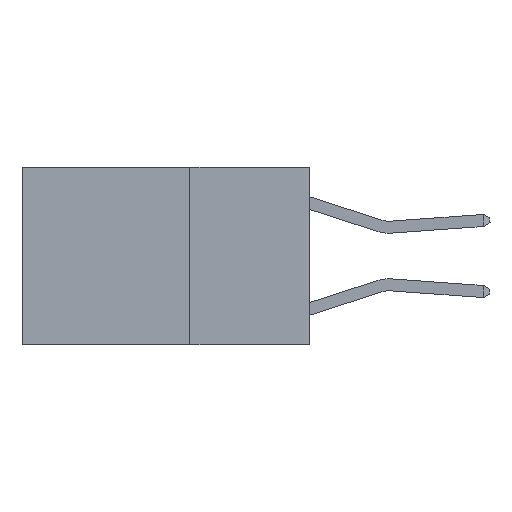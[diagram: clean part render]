
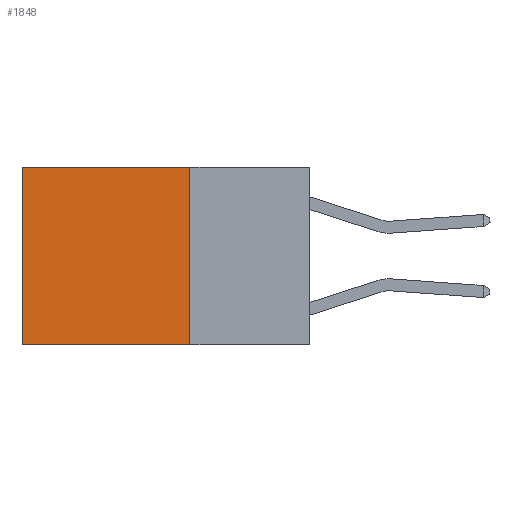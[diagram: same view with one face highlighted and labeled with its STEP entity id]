
A CAD part, left-side view. The second image highlights one B-rep face of the part: STEP entity #1848.
In plain terms, the highlighted planar face has unit normal (-1, 0, 0).
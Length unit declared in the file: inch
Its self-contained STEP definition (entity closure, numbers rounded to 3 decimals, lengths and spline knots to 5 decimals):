
#66 = LINE ( 'NONE', #4859, #17394 ) ;
#236 = LINE ( 'NONE', #1767, #18841 ) ;
#799 = CARTESIAN_POINT ( 'NONE',  ( 0.2625, 0.25, 0. ) ) ;
#1332 = FACE_OUTER_BOUND ( 'NONE', #15989, .T. ) ;
#1666 = ORIENTED_EDGE ( 'NONE', *, *, #2875, .T. ) ;
#1767 = CARTESIAN_POINT ( 'NONE',  ( 0.2625, 0.6, 0. ) ) ;
#1848 = ADVANCED_FACE ( 'NONE', ( #1332 ), #17925, .F. ) ;
#2875 = EDGE_CURVE ( 'NONE', #9417, #7907, #236, .T. ) ;
#4420 = DIRECTION ( 'NONE',  ( 0., 1., 0. ) ) ;
#4859 = CARTESIAN_POINT ( 'NONE',  ( 0.2625, 0.25, -0.37 ) ) ;
#4916 = CARTESIAN_POINT ( 'NONE',  ( 0.2625, 0.25, 0. ) ) ;
#5682 = CARTESIAN_POINT ( 'NONE',  ( 0.2625, 0.6, -0.37 ) ) ;
#5808 = VERTEX_POINT ( 'NONE', #13009 ) ;
#6029 = LINE ( 'NONE', #12667, #20225 ) ;
#6372 = VECTOR ( 'NONE', #18154, 39.37008 ) ;
#6512 = VERTEX_POINT ( 'NONE', #799 ) ;
#6969 = ORIENTED_EDGE ( 'NONE', *, *, #7077, .F. ) ;
#7077 = EDGE_CURVE ( 'NONE', #5808, #7907, #66, .T. ) ;
#7727 = DIRECTION ( 'NONE',  ( 0., 0., -1. ) ) ;
#7779 = ORIENTED_EDGE ( 'NONE', *, *, #8357, .T. ) ;
#7907 = VERTEX_POINT ( 'NONE', #5682 ) ;
#8357 = EDGE_CURVE ( 'NONE', #6512, #9417, #6029, .T. ) ;
#9125 = AXIS2_PLACEMENT_3D ( 'NONE', #14572, #17601, #7727 ) ;
#9417 = VERTEX_POINT ( 'NONE', #18617 ) ;
#10052 = ORIENTED_EDGE ( 'NONE', *, *, #18466, .F. ) ;
#12667 = CARTESIAN_POINT ( 'NONE',  ( 0.2625, 0.25, 0. ) ) ;
#13009 = CARTESIAN_POINT ( 'NONE',  ( 0.2625, 0.25, -0.37 ) ) ;
#14572 = CARTESIAN_POINT ( 'NONE',  ( 0.2625, 0.25, 0. ) ) ;
#15989 = EDGE_LOOP ( 'NONE', ( #1666, #6969, #10052, #7779 ) ) ;
#16840 = DIRECTION ( 'NONE',  ( 0., 0., -1. ) ) ;
#17394 = VECTOR ( 'NONE', #19730, 39.37008 ) ;
#17601 = DIRECTION ( 'NONE',  ( 1., 0., 0. ) ) ;
#17925 = PLANE ( 'NONE',  #9125 ) ;
#18154 = DIRECTION ( 'NONE',  ( 0., 0., -1. ) ) ;
#18466 = EDGE_CURVE ( 'NONE', #6512, #5808, #21337, .T. ) ;
#18617 = CARTESIAN_POINT ( 'NONE',  ( 0.2625, 0.6, 0. ) ) ;
#18841 = VECTOR ( 'NONE', #16840, 39.37008 ) ;
#19730 = DIRECTION ( 'NONE',  ( 0., 1., 0. ) ) ;
#20225 = VECTOR ( 'NONE', #4420, 39.37008 ) ;
#21337 = LINE ( 'NONE', #4916, #6372 ) ;
